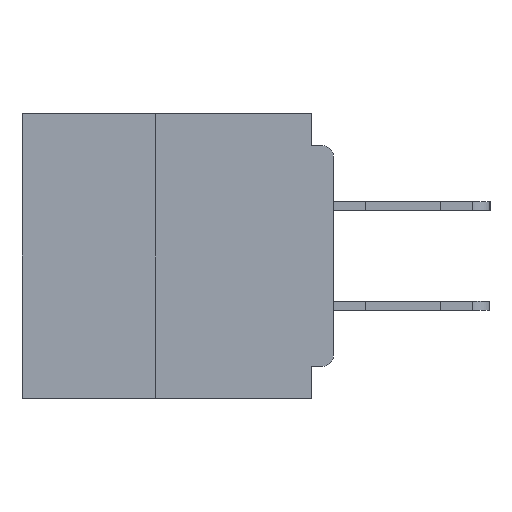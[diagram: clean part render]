
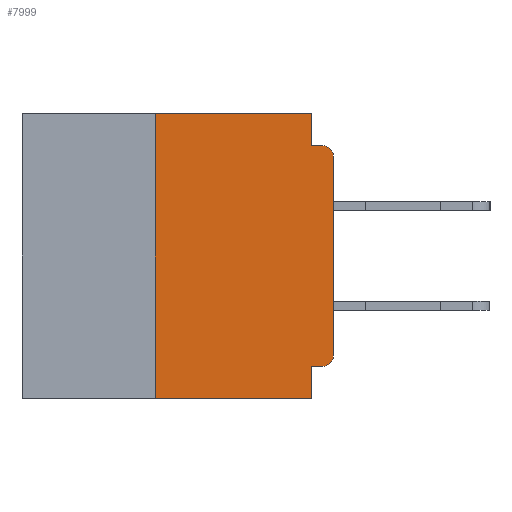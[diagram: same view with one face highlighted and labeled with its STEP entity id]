
A CAD part, left-side view. The second image highlights one B-rep face of the part: STEP entity #7999.
In plain terms, the highlighted planar face has unit normal (-1, 0, 0).
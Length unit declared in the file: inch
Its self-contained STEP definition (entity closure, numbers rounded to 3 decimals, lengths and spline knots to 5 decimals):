
#790 = CARTESIAN_POINT ( 'NONE',  ( 0., 0.031, 0. ) ) ;
#1662 = DIRECTION ( 'NONE',  ( 0., -1., 0. ) ) ;
#2455 = VERTEX_POINT ( 'NONE', #23423 ) ;
#3625 = CARTESIAN_POINT ( 'NONE',  ( 0., 0.25, -0.4 ) ) ;
#3905 = EDGE_CURVE ( 'NONE', #47703, #32544, #24888, .T. ) ;
#5300 = DIRECTION ( 'NONE',  ( 0., 1., 0. ) ) ;
#5729 = ORIENTED_EDGE ( 'NONE', *, *, #10993, .F. ) ;
#7004 = AXIS2_PLACEMENT_3D ( 'NONE', #32288, #14708, #40996 ) ;
#7905 = EDGE_CURVE ( 'NONE', #55479, #20366, #26574, .T. ) ;
#7999 = ADVANCED_FACE ( 'NONE', ( #55647 ), #36676, .F. ) ;
#9615 = EDGE_CURVE ( 'NONE', #27619, #24568, #26343, .T. ) ;
#9793 = CARTESIAN_POINT ( 'NONE',  ( 0., 0.015, -0.355 ) ) ;
#10993 = EDGE_CURVE ( 'NONE', #12191, #17418, #52468, .T. ) ;
#11052 = DIRECTION ( 'NONE',  ( 0., -1., 0. ) ) ;
#11308 = DIRECTION ( 'NONE',  ( 0., 0., 1. ) ) ;
#12191 = VERTEX_POINT ( 'NONE', #44495 ) ;
#12547 = EDGE_CURVE ( 'NONE', #27619, #12191, #41511, .T. ) ;
#13316 = VECTOR ( 'NONE', #45774, 39.37008 ) ;
#14708 = DIRECTION ( 'NONE',  ( 1., 0., 0. ) ) ;
#14725 = VECTOR ( 'NONE', #1662, 39.37008 ) ;
#14892 = LINE ( 'NONE', #55382, #38088 ) ;
#15456 = EDGE_CURVE ( 'NONE', #17418, #47703, #41832, .T. ) ;
#15696 = CIRCLE ( 'NONE', #44044, 0.015 ) ;
#15877 = CARTESIAN_POINT ( 'NONE',  ( 0., 0.031, -0.045 ) ) ;
#16735 = DIRECTION ( 'NONE',  ( 0., 0., 1. ) ) ;
#17418 = VERTEX_POINT ( 'NONE', #26522 ) ;
#18563 = DIRECTION ( 'NONE',  ( -1., 0., 0. ) ) ;
#18708 = VECTOR ( 'NONE', #26853, 39.37008 ) ;
#18987 = CARTESIAN_POINT ( 'NONE',  ( 0., 0.437, -0.4 ) ) ;
#19904 = CARTESIAN_POINT ( 'NONE',  ( 0., 0., 0. ) ) ;
#20366 = VERTEX_POINT ( 'NONE', #40434 ) ;
#20653 = CARTESIAN_POINT ( 'NONE',  ( 0., 0.015, -0.06 ) ) ;
#20784 = VECTOR ( 'NONE', #5300, 39.37008 ) ;
#21591 = LINE ( 'NONE', #19904, #31842 ) ;
#23423 = CARTESIAN_POINT ( 'NONE',  ( 0., 0., -0.06 ) ) ;
#24568 = VERTEX_POINT ( 'NONE', #53684 ) ;
#24888 = LINE ( 'NONE', #46202, #13316 ) ;
#25026 = DIRECTION ( 'NONE',  ( 0., 0., -1. ) ) ;
#25415 = EDGE_CURVE ( 'NONE', #2455, #32544, #15696, .T. ) ;
#25578 = AXIS2_PLACEMENT_3D ( 'NONE', #44564, #18563, #48901 ) ;
#26343 = LINE ( 'NONE', #18987, #14725 ) ;
#26522 = CARTESIAN_POINT ( 'NONE',  ( 0., 0.031, 0. ) ) ;
#26574 = CIRCLE ( 'NONE', #25578, 0.015 ) ;
#26853 = DIRECTION ( 'NONE',  ( 0., 0., -1. ) ) ;
#27619 = VERTEX_POINT ( 'NONE', #34575 ) ;
#27974 = CARTESIAN_POINT ( 'NONE',  ( 0., 0.031, -0.355 ) ) ;
#29562 = DIRECTION ( 'NONE',  ( 0., 0., -1. ) ) ;
#30006 = VECTOR ( 'NONE', #16735, 39.37008 ) ;
#31842 = VECTOR ( 'NONE', #11308, 39.37008 ) ;
#32288 = CARTESIAN_POINT ( 'NONE',  ( 0., 0.437, 0. ) ) ;
#32400 = LINE ( 'NONE', #39939, #20784 ) ;
#32544 = VERTEX_POINT ( 'NONE', #55508 ) ;
#34575 = CARTESIAN_POINT ( 'NONE',  ( 0., 0.25, -0.4 ) ) ;
#36032 = EDGE_CURVE ( 'NONE', #20366, #2455, #21591, .T. ) ;
#36676 = PLANE ( 'NONE',  #7004 ) ;
#37106 = ORIENTED_EDGE ( 'NONE', *, *, #54318, .F. ) ;
#37125 = EDGE_CURVE ( 'NONE', #55479, #46983, #32400, .T. ) ;
#38088 = VECTOR ( 'NONE', #29562, 39.37008 ) ;
#39939 = CARTESIAN_POINT ( 'NONE',  ( 0., 0., -0.355 ) ) ;
#40434 = CARTESIAN_POINT ( 'NONE',  ( 0., 0., -0.34 ) ) ;
#40504 = EDGE_LOOP ( 'NONE', ( #49844, #53880, #55238, #49193, #5729, #41805, #45814, #37106, #52602, #53934 ) ) ;
#40996 = DIRECTION ( 'NONE',  ( 0., 0., -1. ) ) ;
#41013 = VECTOR ( 'NONE', #11052, 39.37008 ) ;
#41511 = LINE ( 'NONE', #3625, #30006 ) ;
#41805 = ORIENTED_EDGE ( 'NONE', *, *, #12547, .F. ) ;
#41832 = LINE ( 'NONE', #790, #18708 ) ;
#44044 = AXIS2_PLACEMENT_3D ( 'NONE', #20653, #50976, #25026 ) ;
#44495 = CARTESIAN_POINT ( 'NONE',  ( 0., 0.25, 0. ) ) ;
#44564 = CARTESIAN_POINT ( 'NONE',  ( 0., 0.015, -0.34 ) ) ;
#45774 = DIRECTION ( 'NONE',  ( 0., -1., 0. ) ) ;
#45814 = ORIENTED_EDGE ( 'NONE', *, *, #9615, .T. ) ;
#46202 = CARTESIAN_POINT ( 'NONE',  ( 0., 0., -0.045 ) ) ;
#46983 = VERTEX_POINT ( 'NONE', #27974 ) ;
#47703 = VERTEX_POINT ( 'NONE', #15877 ) ;
#48901 = DIRECTION ( 'NONE',  ( 0., 0., -1. ) ) ;
#49193 = ORIENTED_EDGE ( 'NONE', *, *, #15456, .F. ) ;
#49844 = ORIENTED_EDGE ( 'NONE', *, *, #36032, .T. ) ;
#50976 = DIRECTION ( 'NONE',  ( -1., 0., 0. ) ) ;
#52468 = LINE ( 'NONE', #54464, #41013 ) ;
#52602 = ORIENTED_EDGE ( 'NONE', *, *, #37125, .F. ) ;
#53684 = CARTESIAN_POINT ( 'NONE',  ( 0., 0.031, -0.4 ) ) ;
#53880 = ORIENTED_EDGE ( 'NONE', *, *, #25415, .T. ) ;
#53934 = ORIENTED_EDGE ( 'NONE', *, *, #7905, .T. ) ;
#54318 = EDGE_CURVE ( 'NONE', #46983, #24568, #14892, .T. ) ;
#54464 = CARTESIAN_POINT ( 'NONE',  ( 0., 0.437, 0. ) ) ;
#55238 = ORIENTED_EDGE ( 'NONE', *, *, #3905, .F. ) ;
#55382 = CARTESIAN_POINT ( 'NONE',  ( 0., 0.031, -0.4 ) ) ;
#55479 = VERTEX_POINT ( 'NONE', #9793 ) ;
#55508 = CARTESIAN_POINT ( 'NONE',  ( 0., 0.015, -0.045 ) ) ;
#55647 = FACE_OUTER_BOUND ( 'NONE', #40504, .T. ) ;
